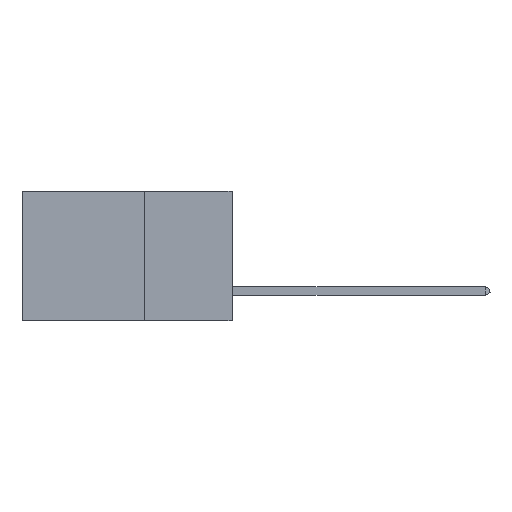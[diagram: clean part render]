
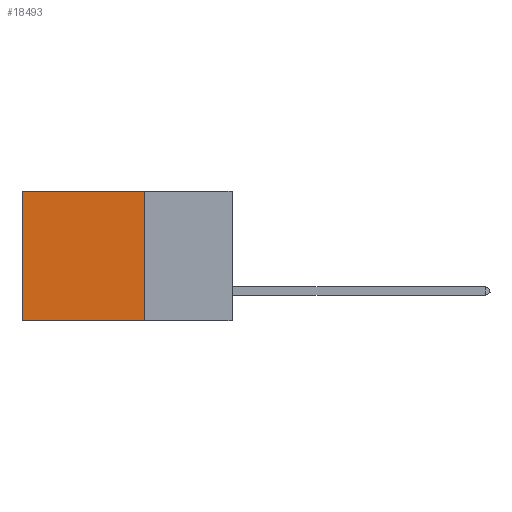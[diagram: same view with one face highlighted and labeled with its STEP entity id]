
A CAD part, left-side view. The second image highlights one B-rep face of the part: STEP entity #18493.
In plain terms, the highlighted planar face has unit normal (-1, 0, 0).
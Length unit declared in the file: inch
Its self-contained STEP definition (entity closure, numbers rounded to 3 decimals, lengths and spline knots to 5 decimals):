
#345 = VERTEX_POINT ( 'NONE', #3939 ) ;
#616 = CARTESIAN_POINT ( 'NONE',  ( 0.2875, 0.6, 0. ) ) ;
#1309 = DIRECTION ( 'NONE',  ( 0., 1., 0. ) ) ;
#1422 = VERTEX_POINT ( 'NONE', #9895 ) ;
#2101 = VERTEX_POINT ( 'NONE', #20113 ) ;
#3816 = VECTOR ( 'NONE', #1309, 39.37008 ) ;
#3836 = ORIENTED_EDGE ( 'NONE', *, *, #19869, .F. ) ;
#3939 = CARTESIAN_POINT ( 'NONE',  ( 0.2875, 0.6, -0.37 ) ) ;
#3964 = LINE ( 'NONE', #15513, #21401 ) ;
#4383 = LINE ( 'NONE', #8296, #3816 ) ;
#4524 = CARTESIAN_POINT ( 'NONE',  ( 0.2875, 0.25, 0. ) ) ;
#5761 = PLANE ( 'NONE',  #9933 ) ;
#6165 = EDGE_CURVE ( 'NONE', #13692, #345, #6829, .T. ) ;
#6796 = DIRECTION ( 'NONE',  ( 0., 1., 0. ) ) ;
#6829 = LINE ( 'NONE', #19741, #14280 ) ;
#8296 = CARTESIAN_POINT ( 'NONE',  ( 0.2875, 0.25, -0.37 ) ) ;
#9165 = DIRECTION ( 'NONE',  ( 0., 0., -1. ) ) ;
#9460 = CARTESIAN_POINT ( 'NONE',  ( 0.2875, 0.25, 0. ) ) ;
#9844 = LINE ( 'NONE', #4524, #18423 ) ;
#9895 = CARTESIAN_POINT ( 'NONE',  ( 0.2875, 0.25, -0.37 ) ) ;
#9933 = AXIS2_PLACEMENT_3D ( 'NONE', #9460, #16342, #21643 ) ;
#11067 = FACE_OUTER_BOUND ( 'NONE', #16733, .T. ) ;
#11544 = ORIENTED_EDGE ( 'NONE', *, *, #6165, .T. ) ;
#11763 = ORIENTED_EDGE ( 'NONE', *, *, #15779, .F. ) ;
#13692 = VERTEX_POINT ( 'NONE', #616 ) ;
#14280 = VECTOR ( 'NONE', #9165, 39.37008 ) ;
#14778 = DIRECTION ( 'NONE',  ( 0., 0., -1. ) ) ;
#15513 = CARTESIAN_POINT ( 'NONE',  ( 0.2875, 0.25, 0. ) ) ;
#15779 = EDGE_CURVE ( 'NONE', #2101, #1422, #9844, .T. ) ;
#16342 = DIRECTION ( 'NONE',  ( 1., 0., 0. ) ) ;
#16617 = EDGE_CURVE ( 'NONE', #2101, #13692, #3964, .T. ) ;
#16733 = EDGE_LOOP ( 'NONE', ( #11544, #3836, #11763, #18971 ) ) ;
#18423 = VECTOR ( 'NONE', #14778, 39.37008 ) ;
#18493 = ADVANCED_FACE ( 'NONE', ( #11067 ), #5761, .F. ) ;
#18971 = ORIENTED_EDGE ( 'NONE', *, *, #16617, .T. ) ;
#19741 = CARTESIAN_POINT ( 'NONE',  ( 0.2875, 0.6, 0. ) ) ;
#19869 = EDGE_CURVE ( 'NONE', #1422, #345, #4383, .T. ) ;
#20113 = CARTESIAN_POINT ( 'NONE',  ( 0.2875, 0.25, 0. ) ) ;
#21401 = VECTOR ( 'NONE', #6796, 39.37008 ) ;
#21643 = DIRECTION ( 'NONE',  ( 0., 0., -1. ) ) ;
